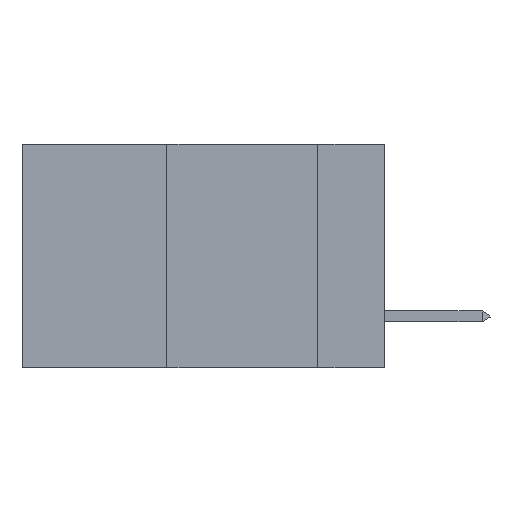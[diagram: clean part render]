
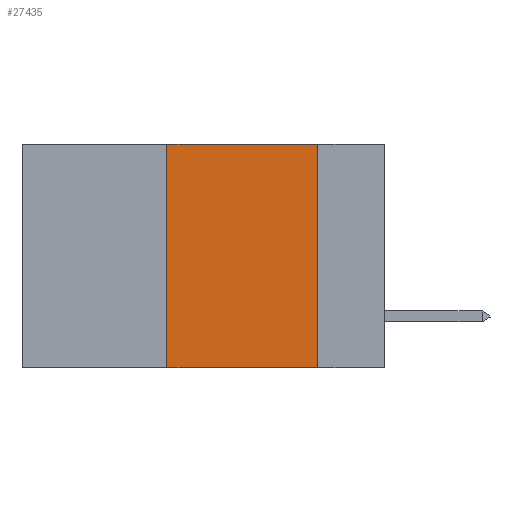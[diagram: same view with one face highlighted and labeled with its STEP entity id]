
A CAD part, left-side view. The second image highlights one B-rep face of the part: STEP entity #27435.
In plain terms, the highlighted planar face has unit normal (-1, 0, 0).
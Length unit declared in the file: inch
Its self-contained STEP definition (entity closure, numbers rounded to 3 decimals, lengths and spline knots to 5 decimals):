
#3339 = PLANE ( 'NONE',  #35796 ) ;
#3691 = CARTESIAN_POINT ( 'NONE',  ( 0., 0.6, 0. ) ) ;
#7055 = ORIENTED_EDGE ( 'NONE', *, *, #15400, .F. ) ;
#10248 = VECTOR ( 'NONE', #15843, 39.37008 ) ;
#13080 = ORIENTED_EDGE ( 'NONE', *, *, #16862, .T. ) ;
#13547 = VERTEX_POINT ( 'NONE', #19136 ) ;
#13753 = VERTEX_POINT ( 'NONE', #20888 ) ;
#14513 = VERTEX_POINT ( 'NONE', #49082 ) ;
#15400 = EDGE_CURVE ( 'NONE', #13753, #13547, #23760, .T. ) ;
#15622 = CARTESIAN_POINT ( 'NONE',  ( 0., 0.11, 0. ) ) ;
#15843 = DIRECTION ( 'NONE',  ( 0., -1., 0. ) ) ;
#16862 = EDGE_CURVE ( 'NONE', #37803, #13547, #39820, .T. ) ;
#19136 = CARTESIAN_POINT ( 'NONE',  ( 0., 0.11, -0.37 ) ) ;
#20888 = CARTESIAN_POINT ( 'NONE',  ( 0., 0.11, 0. ) ) ;
#21255 = CARTESIAN_POINT ( 'NONE',  ( 0., 0.6, -0.37 ) ) ;
#21372 = LINE ( 'NONE', #31886, #25677 ) ;
#22415 = VECTOR ( 'NONE', #28906, 39.37008 ) ;
#22506 = VECTOR ( 'NONE', #43949, 39.37008 ) ;
#23538 = DIRECTION ( 'NONE',  ( 0., 0., 1. ) ) ;
#23760 = LINE ( 'NONE', #15622, #22506 ) ;
#24654 = FACE_OUTER_BOUND ( 'NONE', #34388, .T. ) ;
#25677 = VECTOR ( 'NONE', #23538, 39.37008 ) ;
#25936 = CARTESIAN_POINT ( 'NONE',  ( 0., 0.36, -0.37 ) ) ;
#27435 = ADVANCED_FACE ( 'NONE', ( #24654 ), #3339, .F. ) ;
#28041 = CARTESIAN_POINT ( 'NONE',  ( 0., 0.6, 0. ) ) ;
#28906 = DIRECTION ( 'NONE',  ( 0., -1., 0. ) ) ;
#31211 = DIRECTION ( 'NONE',  ( 0., 0., -1. ) ) ;
#31886 = CARTESIAN_POINT ( 'NONE',  ( 0., 0.36, 0. ) ) ;
#33820 = ORIENTED_EDGE ( 'NONE', *, *, #47765, .F. ) ;
#34388 = EDGE_LOOP ( 'NONE', ( #7055, #45457, #33820, #13080 ) ) ;
#35796 = AXIS2_PLACEMENT_3D ( 'NONE', #3691, #51347, #31211 ) ;
#37803 = VERTEX_POINT ( 'NONE', #25936 ) ;
#39820 = LINE ( 'NONE', #21255, #22415 ) ;
#43949 = DIRECTION ( 'NONE',  ( 0., 0., -1. ) ) ;
#45101 = LINE ( 'NONE', #28041, #10248 ) ;
#45457 = ORIENTED_EDGE ( 'NONE', *, *, #46598, .F. ) ;
#46598 = EDGE_CURVE ( 'NONE', #14513, #13753, #45101, .T. ) ;
#47765 = EDGE_CURVE ( 'NONE', #37803, #14513, #21372, .T. ) ;
#49082 = CARTESIAN_POINT ( 'NONE',  ( 0., 0.36, 0. ) ) ;
#51347 = DIRECTION ( 'NONE',  ( 1., 0., 0. ) ) ;
